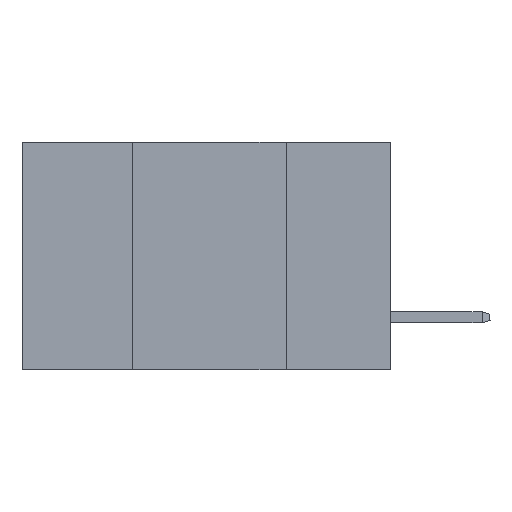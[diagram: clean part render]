
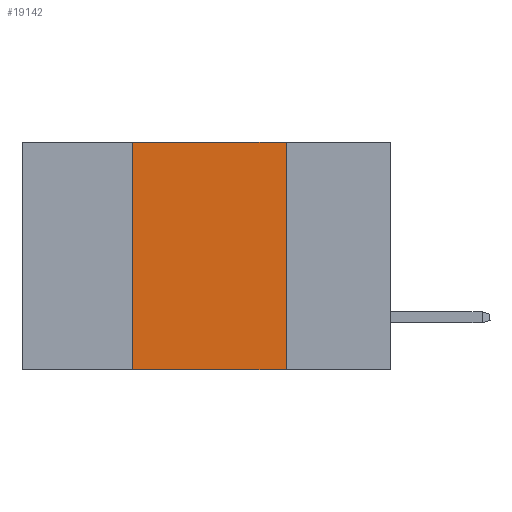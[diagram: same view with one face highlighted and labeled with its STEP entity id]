
A CAD part, left-side view. The second image highlights one B-rep face of the part: STEP entity #19142.
In plain terms, the highlighted planar face has unit normal (-1, 0, 0).
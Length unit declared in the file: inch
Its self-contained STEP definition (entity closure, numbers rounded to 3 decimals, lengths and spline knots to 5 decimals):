
#2970 = FACE_OUTER_BOUND ( 'NONE', #9105, .T. ) ;
#3391 = PLANE ( 'NONE',  #20423 ) ;
#3392 = CARTESIAN_POINT ( 'NONE',  ( 0., 0.42, 0. ) ) ;
#3668 = CARTESIAN_POINT ( 'NONE',  ( 0., 0.17, 0. ) ) ;
#3992 = VERTEX_POINT ( 'NONE', #18861 ) ;
#4540 = ORIENTED_EDGE ( 'NONE', *, *, #18595, .F. ) ;
#5574 = LINE ( 'NONE', #7083, #17961 ) ;
#5714 = VERTEX_POINT ( 'NONE', #20952 ) ;
#6068 = CARTESIAN_POINT ( 'NONE',  ( 0., 0.42, 0. ) ) ;
#7083 = CARTESIAN_POINT ( 'NONE',  ( 0., 0.6, -0.37 ) ) ;
#7236 = DIRECTION ( 'NONE',  ( 0., 0., -1. ) ) ;
#8581 = ORIENTED_EDGE ( 'NONE', *, *, #20226, .F. ) ;
#9105 = EDGE_LOOP ( 'NONE', ( #4540, #8581, #19952, #22029 ) ) ;
#9650 = VERTEX_POINT ( 'NONE', #3392 ) ;
#10711 = LINE ( 'NONE', #3668, #19669 ) ;
#10867 = LINE ( 'NONE', #6068, #13988 ) ;
#11610 = EDGE_CURVE ( 'NONE', #5714, #3992, #5574, .T. ) ;
#11611 = DIRECTION ( 'NONE',  ( 0., 0., -1. ) ) ;
#13988 = VECTOR ( 'NONE', #23328, 39.37008 ) ;
#15159 = CARTESIAN_POINT ( 'NONE',  ( 0., 0.17, 0. ) ) ;
#17107 = VECTOR ( 'NONE', #20841, 39.37008 ) ;
#17198 = CARTESIAN_POINT ( 'NONE',  ( 0., 0.6, 0. ) ) ;
#17405 = LINE ( 'NONE', #17198, #17107 ) ;
#17961 = VECTOR ( 'NONE', #19724, 39.37008 ) ;
#18595 = EDGE_CURVE ( 'NONE', #25355, #3992, #10711, .T. ) ;
#18861 = CARTESIAN_POINT ( 'NONE',  ( 0., 0.17, -0.37 ) ) ;
#19142 = ADVANCED_FACE ( 'NONE', ( #2970 ), #3391, .F. ) ;
#19669 = VECTOR ( 'NONE', #11611, 39.37008 ) ;
#19724 = DIRECTION ( 'NONE',  ( 0., -1., 0. ) ) ;
#19952 = ORIENTED_EDGE ( 'NONE', *, *, #20968, .F. ) ;
#20226 = EDGE_CURVE ( 'NONE', #9650, #25355, #17405, .T. ) ;
#20423 = AXIS2_PLACEMENT_3D ( 'NONE', #25363, #25441, #7236 ) ;
#20841 = DIRECTION ( 'NONE',  ( 0., -1., 0. ) ) ;
#20952 = CARTESIAN_POINT ( 'NONE',  ( 0., 0.42, -0.37 ) ) ;
#20968 = EDGE_CURVE ( 'NONE', #5714, #9650, #10867, .T. ) ;
#22029 = ORIENTED_EDGE ( 'NONE', *, *, #11610, .T. ) ;
#23328 = DIRECTION ( 'NONE',  ( 0., 0., 1. ) ) ;
#25355 = VERTEX_POINT ( 'NONE', #15159 ) ;
#25363 = CARTESIAN_POINT ( 'NONE',  ( 0., 0.6, 0. ) ) ;
#25441 = DIRECTION ( 'NONE',  ( 1., 0., 0. ) ) ;
